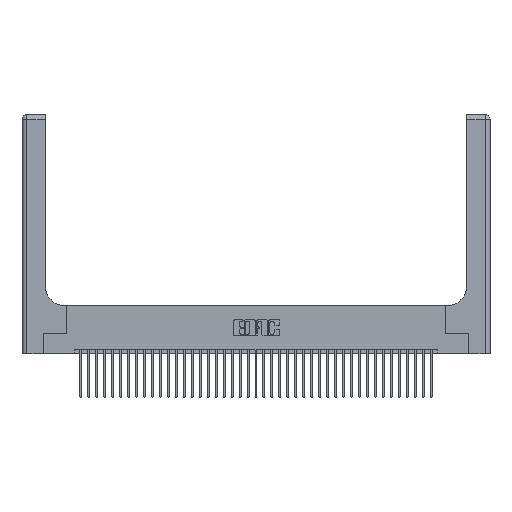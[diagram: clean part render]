
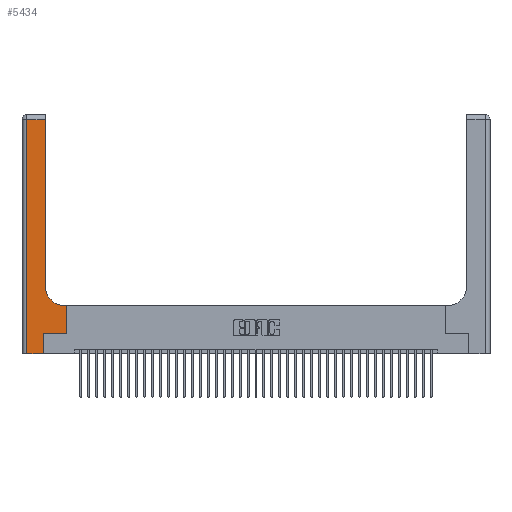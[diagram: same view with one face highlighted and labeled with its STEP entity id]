
A CAD part, top view. The second image highlights one B-rep face of the part: STEP entity #5434.
In plain terms, the highlighted planar face has unit normal (0, 0, 1).
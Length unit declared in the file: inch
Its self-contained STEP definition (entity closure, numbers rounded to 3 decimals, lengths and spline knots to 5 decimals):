
#576 = ORIENTED_EDGE ( 'NONE', *, *, #18816, .T. ) ;
#628 = VECTOR ( 'NONE', #19730, 39.37008 ) ;
#723 = LINE ( 'NONE', #15102, #32694 ) ;
#979 = DIRECTION ( 'NONE',  ( 0., -1., 0. ) ) ;
#1643 = LINE ( 'NONE', #11262, #30653 ) ;
#2511 = VECTOR ( 'NONE', #979, 39.37008 ) ;
#2637 = VERTEX_POINT ( 'NONE', #9568 ) ;
#2702 = AXIS2_PLACEMENT_3D ( 'NONE', #16083, #31744, #29038 ) ;
#3215 = ORIENTED_EDGE ( 'NONE', *, *, #26436, .T. ) ;
#5434 = ADVANCED_FACE ( 'NONE', ( #15846 ), #19444, .F. ) ;
#5465 = ORIENTED_EDGE ( 'NONE', *, *, #9622, .T. ) ;
#5749 = VECTOR ( 'NONE', #19033, 39.37008 ) ;
#6243 = VERTEX_POINT ( 'NONE', #12331 ) ;
#6586 = CARTESIAN_POINT ( 'NONE',  ( 0., 2.94, 0.37 ) ) ;
#7550 = CARTESIAN_POINT ( 'NONE',  ( 0.2915, 2.94, 0.37 ) ) ;
#8482 = CARTESIAN_POINT ( 'NONE',  ( 0.5415, 0.6, 0.37 ) ) ;
#9568 = CARTESIAN_POINT ( 'NONE',  ( 0.06, 2.94, 0.37 ) ) ;
#9622 = EDGE_CURVE ( 'NONE', #29836, #24825, #15107, .T. ) ;
#11150 = CARTESIAN_POINT ( 'NONE',  ( 0.269, 0., 0.37 ) ) ;
#11262 = CARTESIAN_POINT ( 'NONE',  ( 0.269, 0., 0.37 ) ) ;
#11525 = ORIENTED_EDGE ( 'NONE', *, *, #14903, .T. ) ;
#11715 = CARTESIAN_POINT ( 'NONE',  ( 0.2915, 0.6, 0.37 ) ) ;
#12331 = CARTESIAN_POINT ( 'NONE',  ( 0.269, 0.25, 0.37 ) ) ;
#13725 = CARTESIAN_POINT ( 'NONE',  ( 0.2915, 0.85, 0.37 ) ) ;
#13751 = LINE ( 'NONE', #6586, #37416 ) ;
#13933 = VECTOR ( 'NONE', #39858, 39.37008 ) ;
#13965 = LINE ( 'NONE', #25239, #5749 ) ;
#13979 = EDGE_CURVE ( 'NONE', #24825, #22133, #13965, .T. ) ;
#14293 = LINE ( 'NONE', #31483, #628 ) ;
#14597 = CARTESIAN_POINT ( 'NONE',  ( 0.5415, 0.85, 0.37 ) ) ;
#14903 = EDGE_CURVE ( 'NONE', #20486, #29836, #35686, .T. ) ;
#15096 = LINE ( 'NONE', #34377, #37315 ) ;
#15102 = CARTESIAN_POINT ( 'NONE',  ( 0.269, 0.25, 0.37 ) ) ;
#15107 = CIRCLE ( 'NONE', #32257, 0.25 ) ;
#15846 = FACE_OUTER_BOUND ( 'NONE', #18485, .T. ) ;
#16083 = CARTESIAN_POINT ( 'NONE',  ( 0., 3., 0.37 ) ) ;
#16211 = VERTEX_POINT ( 'NONE', #34806 ) ;
#16817 = EDGE_CURVE ( 'NONE', #24841, #6243, #1643, .T. ) ;
#17151 = EDGE_CURVE ( 'NONE', #22133, #2637, #13751, .T. ) ;
#18307 = CARTESIAN_POINT ( 'NONE',  ( 0.5585, 0.25, 0.37 ) ) ;
#18485 = EDGE_LOOP ( 'NONE', ( #38748, #25121, #576, #23155, #36922, #33824, #3215, #11525, #5465 ) ) ;
#18816 = EDGE_CURVE ( 'NONE', #2637, #16211, #34396, .T. ) ;
#19033 = DIRECTION ( 'NONE',  ( 0., 1., 0. ) ) ;
#19444 = PLANE ( 'NONE',  #2702 ) ;
#19730 = DIRECTION ( 'NONE',  ( 0., 1., 0. ) ) ;
#20389 = DIRECTION ( 'NONE',  ( 1., 0., 0. ) ) ;
#20486 = VERTEX_POINT ( 'NONE', #25766 ) ;
#22133 = VERTEX_POINT ( 'NONE', #7550 ) ;
#22173 = VERTEX_POINT ( 'NONE', #18307 ) ;
#23155 = ORIENTED_EDGE ( 'NONE', *, *, #35020, .T. ) ;
#24825 = VERTEX_POINT ( 'NONE', #13725 ) ;
#24841 = VERTEX_POINT ( 'NONE', #11150 ) ;
#25121 = ORIENTED_EDGE ( 'NONE', *, *, #17151, .T. ) ;
#25239 = CARTESIAN_POINT ( 'NONE',  ( 0.2915, 3., 0.37 ) ) ;
#25331 = CARTESIAN_POINT ( 'NONE',  ( 0.06, 3., 0.37 ) ) ;
#25766 = CARTESIAN_POINT ( 'NONE',  ( 0.5585, 0.6, 0.37 ) ) ;
#26436 = EDGE_CURVE ( 'NONE', #22173, #20486, #14293, .T. ) ;
#28415 = DIRECTION ( 'NONE',  ( 1., 0., 0. ) ) ;
#29038 = DIRECTION ( 'NONE',  ( -1., 0., 0. ) ) ;
#29836 = VERTEX_POINT ( 'NONE', #8482 ) ;
#30653 = VECTOR ( 'NONE', #35457, 39.37008 ) ;
#31483 = CARTESIAN_POINT ( 'NONE',  ( 0.5585, 0.25, 0.37 ) ) ;
#31744 = DIRECTION ( 'NONE',  ( 0., 0., -1. ) ) ;
#32257 = AXIS2_PLACEMENT_3D ( 'NONE', #14597, #35812, #20389 ) ;
#32694 = VECTOR ( 'NONE', #33053, 39.37008 ) ;
#33053 = DIRECTION ( 'NONE',  ( 1., 0., 0. ) ) ;
#33824 = ORIENTED_EDGE ( 'NONE', *, *, #38736, .T. ) ;
#34377 = CARTESIAN_POINT ( 'NONE',  ( 0., 0., 0.37 ) ) ;
#34396 = LINE ( 'NONE', #25331, #2511 ) ;
#34806 = CARTESIAN_POINT ( 'NONE',  ( 0.06, 0., 0.37 ) ) ;
#35020 = EDGE_CURVE ( 'NONE', #16211, #24841, #15096, .T. ) ;
#35457 = DIRECTION ( 'NONE',  ( 0., 1., 0. ) ) ;
#35686 = LINE ( 'NONE', #11715, #13933 ) ;
#35812 = DIRECTION ( 'NONE',  ( 0., 0., -1. ) ) ;
#36922 = ORIENTED_EDGE ( 'NONE', *, *, #16817, .T. ) ;
#37315 = VECTOR ( 'NONE', #28415, 39.37008 ) ;
#37416 = VECTOR ( 'NONE', #37673, 39.37008 ) ;
#37673 = DIRECTION ( 'NONE',  ( -1., 0., 0. ) ) ;
#38736 = EDGE_CURVE ( 'NONE', #6243, #22173, #723, .T. ) ;
#38748 = ORIENTED_EDGE ( 'NONE', *, *, #13979, .T. ) ;
#39858 = DIRECTION ( 'NONE',  ( -1., 0., 0. ) ) ;
